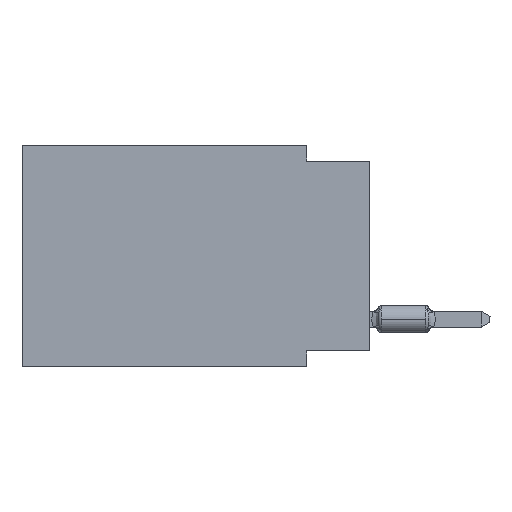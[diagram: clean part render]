
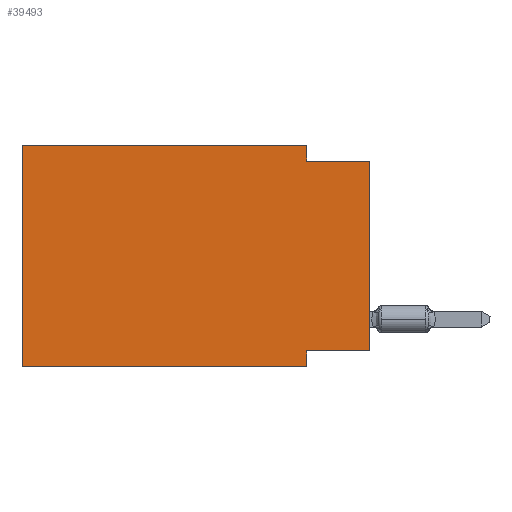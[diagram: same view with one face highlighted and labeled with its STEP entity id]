
A CAD part, left-side view. The second image highlights one B-rep face of the part: STEP entity #39493.
In plain terms, the highlighted planar face has unit normal (-1, 0, 0).
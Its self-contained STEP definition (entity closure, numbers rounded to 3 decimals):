
#801 = CARTESIAN_POINT ( 'NONE',  ( 0., 13.97, -8.89 ) ) ;
#830 = EDGE_CURVE ( 'NONE', #43092, #47399, #44876, .T. ) ;
#1471 = VECTOR ( 'NONE', #26152, 1000. ) ;
#3987 = DIRECTION ( 'NONE',  ( 0., 1., 0. ) ) ;
#4611 = LINE ( 'NONE', #22636, #48123 ) ;
#4640 = VERTEX_POINT ( 'NONE', #43076 ) ;
#6349 = CARTESIAN_POINT ( 'NONE',  ( 0., 2.54, -0.635 ) ) ;
#7165 = CARTESIAN_POINT ( 'NONE',  ( 0., 2.54, -8.255 ) ) ;
#7783 = CARTESIAN_POINT ( 'NONE',  ( 0., 13.97, 0. ) ) ;
#8028 = DIRECTION ( 'NONE',  ( 1., 0., 0. ) ) ;
#8630 = DIRECTION ( 'NONE',  ( 0., 0., 1. ) ) ;
#8904 = ORIENTED_EDGE ( 'NONE', *, *, #830, .F. ) ;
#9430 = LINE ( 'NONE', #20872, #40982 ) ;
#9983 = LINE ( 'NONE', #28978, #18599 ) ;
#10117 = DIRECTION ( 'NONE',  ( 0., -1., 0. ) ) ;
#10448 = AXIS2_PLACEMENT_3D ( 'NONE', #7783, #8028, #44540 ) ;
#11313 = ORIENTED_EDGE ( 'NONE', *, *, #44679, .F. ) ;
#12996 = LINE ( 'NONE', #27848, #29967 ) ;
#13895 = VERTEX_POINT ( 'NONE', #801 ) ;
#15080 = CARTESIAN_POINT ( 'NONE',  ( 0., 0., -0.635 ) ) ;
#15991 = VECTOR ( 'NONE', #3987, 1000. ) ;
#18599 = VECTOR ( 'NONE', #21916, 1000. ) ;
#18849 = ORIENTED_EDGE ( 'NONE', *, *, #21814, .T. ) ;
#18921 = EDGE_LOOP ( 'NONE', ( #41646, #23795, #22116, #46500, #22365, #18849, #11313, #8904 ) ) ;
#20011 = VERTEX_POINT ( 'NONE', #15080 ) ;
#20872 = CARTESIAN_POINT ( 'NONE',  ( 0., 0., -0.635 ) ) ;
#21351 = DIRECTION ( 'NONE',  ( 0., -1., 0. ) ) ;
#21814 = EDGE_CURVE ( 'NONE', #13895, #41387, #38844, .T. ) ;
#21916 = DIRECTION ( 'NONE',  ( 0., -1., 0. ) ) ;
#22116 = ORIENTED_EDGE ( 'NONE', *, *, #27317, .F. ) ;
#22365 = ORIENTED_EDGE ( 'NONE', *, *, #40356, .F. ) ;
#22636 = CARTESIAN_POINT ( 'NONE',  ( 0., 2.54, -8.89 ) ) ;
#23222 = CARTESIAN_POINT ( 'NONE',  ( 0., 0., 0. ) ) ;
#23795 = ORIENTED_EDGE ( 'NONE', *, *, #33182, .F. ) ;
#26152 = DIRECTION ( 'NONE',  ( 0., 0., 1. ) ) ;
#26771 = PLANE ( 'NONE',  #10448 ) ;
#27317 = EDGE_CURVE ( 'NONE', #4640, #39363, #35499, .T. ) ;
#27848 = CARTESIAN_POINT ( 'NONE',  ( 0., 13.97, 0. ) ) ;
#28978 = CARTESIAN_POINT ( 'NONE',  ( 0., 13.97, 0. ) ) ;
#29697 = DIRECTION ( 'NONE',  ( 0., 0., -1. ) ) ;
#29967 = VECTOR ( 'NONE', #8630, 1000. ) ;
#30281 = LINE ( 'NONE', #23222, #1471 ) ;
#32295 = CARTESIAN_POINT ( 'NONE',  ( 0., 0., -8.255 ) ) ;
#32937 = CARTESIAN_POINT ( 'NONE',  ( 0., 13.97, 0. ) ) ;
#33182 = EDGE_CURVE ( 'NONE', #39363, #20011, #9430, .T. ) ;
#33332 = FACE_OUTER_BOUND ( 'NONE', #18921, .T. ) ;
#34823 = VERTEX_POINT ( 'NONE', #32937 ) ;
#35396 = VECTOR ( 'NONE', #10117, 1000. ) ;
#35401 = VECTOR ( 'NONE', #35730, 1000. ) ;
#35499 = LINE ( 'NONE', #36209, #35401 ) ;
#35730 = DIRECTION ( 'NONE',  ( 0., 0., -1. ) ) ;
#36209 = CARTESIAN_POINT ( 'NONE',  ( 0., 2.54, 0. ) ) ;
#37077 = CARTESIAN_POINT ( 'NONE',  ( 0., 0., -8.255 ) ) ;
#38844 = LINE ( 'NONE', #39322, #35396 ) ;
#39322 = CARTESIAN_POINT ( 'NONE',  ( 0., 13.97, -8.89 ) ) ;
#39363 = VERTEX_POINT ( 'NONE', #6349 ) ;
#39493 = ADVANCED_FACE ( 'NONE', ( #33332 ), #26771, .F. ) ;
#40356 = EDGE_CURVE ( 'NONE', #13895, #34823, #12996, .T. ) ;
#40982 = VECTOR ( 'NONE', #21351, 1000. ) ;
#41387 = VERTEX_POINT ( 'NONE', #46894 ) ;
#41646 = ORIENTED_EDGE ( 'NONE', *, *, #43739, .T. ) ;
#43076 = CARTESIAN_POINT ( 'NONE',  ( 0., 2.54, 0. ) ) ;
#43092 = VERTEX_POINT ( 'NONE', #32295 ) ;
#43739 = EDGE_CURVE ( 'NONE', #43092, #20011, #30281, .T. ) ;
#44484 = EDGE_CURVE ( 'NONE', #34823, #4640, #9983, .T. ) ;
#44540 = DIRECTION ( 'NONE',  ( 0., 0., -1. ) ) ;
#44679 = EDGE_CURVE ( 'NONE', #47399, #41387, #4611, .T. ) ;
#44876 = LINE ( 'NONE', #37077, #15991 ) ;
#46500 = ORIENTED_EDGE ( 'NONE', *, *, #44484, .F. ) ;
#46894 = CARTESIAN_POINT ( 'NONE',  ( 0., 2.54, -8.89 ) ) ;
#47399 = VERTEX_POINT ( 'NONE', #7165 ) ;
#48123 = VECTOR ( 'NONE', #29697, 1000. ) ;
